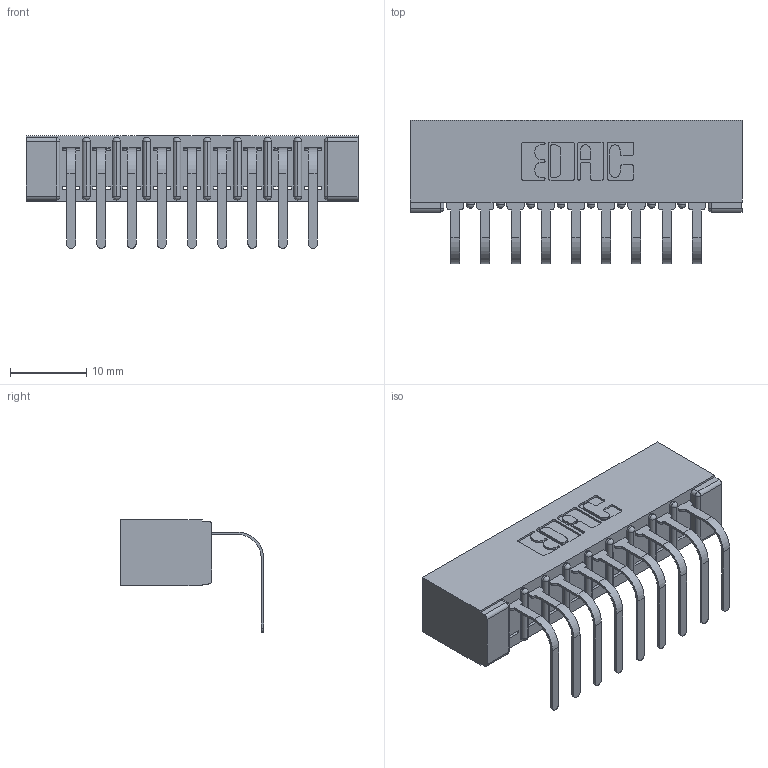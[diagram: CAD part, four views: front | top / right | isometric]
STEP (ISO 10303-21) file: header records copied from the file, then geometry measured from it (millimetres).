
FILE_DESCRIPTION (( 'STEP AP203' ), '1' );
FILE_NAME ('357-009-458-101.STEP', '2022-07-19T00:09:16', ( '' ), ( '' ), 'SwSTEP 2.0', 'SolidWorks 2020', '' );
FILE_SCHEMA (( 'CONFIG_CONTROL_DESIGN' ));
Length unit declared in the file: inch
Products named in the file (3): 357-009-458-101; 307 Part_No Mounting Lugs; 307-290-001_558 - 2 (Single)
Assembly tree (10 placements, depth 2):
  357-009-458-101
    307 Part_No Mounting Lugs
    307-290-001_558 - 2 (Single)  x9
Bounding box: 43.54 x 18.78 x 14.81 mm (x, y, z)
Volume: 3016.8 mm3; surface area: 4724.6 mm2
Topology: 10 solids, 10 shells, 660 faces, 1865 edges, 1202 vertices
Faces by surface type: plane 417, cylinder 223, sphere 20
Entity records: 11610 total; most frequent: CARTESIAN_POINT 1944, ORIENTED_EDGE 1930, DIRECTION 1909, EDGE_CURVE 965, VECTOR 727, LINE 727, VERTEX_POINT 626, AXIS2_PLACEMENT_3D 591
